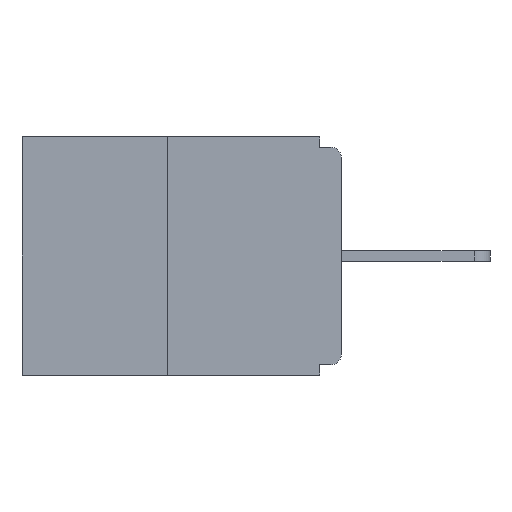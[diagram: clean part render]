
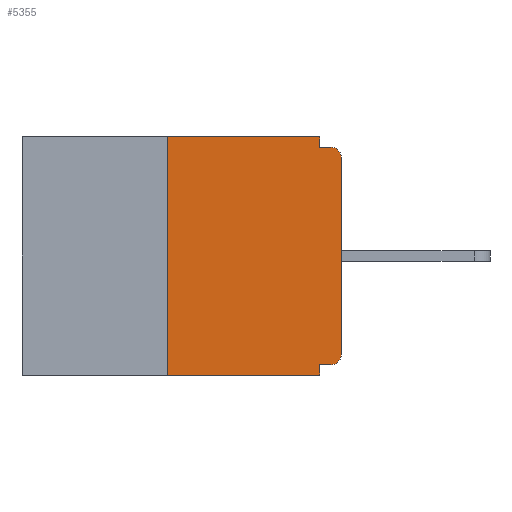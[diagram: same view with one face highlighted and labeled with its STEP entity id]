
A CAD part, left-side view. The second image highlights one B-rep face of the part: STEP entity #5355.
In plain terms, the highlighted planar face has unit normal (-1, 0, 0).
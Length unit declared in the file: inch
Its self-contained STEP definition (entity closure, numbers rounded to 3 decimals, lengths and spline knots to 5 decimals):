
#325 = ORIENTED_EDGE ( 'NONE', *, *, #5950, .T. ) ;
#400 = VERTEX_POINT ( 'NONE', #7091 ) ;
#432 = ORIENTED_EDGE ( 'NONE', *, *, #6960, .F. ) ;
#612 = AXIS2_PLACEMENT_3D ( 'NONE', #7975, #9048, #1179 ) ;
#764 = EDGE_CURVE ( 'NONE', #2450, #3988, #14203, .T. ) ;
#842 = VERTEX_POINT ( 'NONE', #9513 ) ;
#1100 = LINE ( 'NONE', #4835, #7129 ) ;
#1179 = DIRECTION ( 'NONE',  ( 0., 0., -1. ) ) ;
#1227 = DIRECTION ( 'NONE',  ( 0., -1., 0. ) ) ;
#1235 = EDGE_CURVE ( 'NONE', #7766, #1553, #11069, .T. ) ;
#1310 = LINE ( 'NONE', #10430, #7893 ) ;
#1400 = CARTESIAN_POINT ( 'NONE',  ( 0., 0., -0.328 ) ) ;
#1475 = EDGE_CURVE ( 'NONE', #2450, #7743, #1310, .T. ) ;
#1532 = CARTESIAN_POINT ( 'NONE',  ( 0., 0.46, 0. ) ) ;
#1553 = VERTEX_POINT ( 'NONE', #8556 ) ;
#1859 = CARTESIAN_POINT ( 'NONE',  ( 0., 0., -0.015 ) ) ;
#2295 = CARTESIAN_POINT ( 'NONE',  ( 0., 0., 0. ) ) ;
#2450 = VERTEX_POINT ( 'NONE', #4748 ) ;
#2460 = EDGE_CURVE ( 'NONE', #3988, #400, #8192, .T. ) ;
#2547 = DIRECTION ( 'NONE',  ( 0., -1., 0. ) ) ;
#3013 = DIRECTION ( 'NONE',  ( 0., -1., 0. ) ) ;
#3094 = EDGE_CURVE ( 'NONE', #842, #6810, #11705, .T. ) ;
#3638 = CARTESIAN_POINT ( 'NONE',  ( 0., 0.031, 0. ) ) ;
#3669 = VERTEX_POINT ( 'NONE', #6268 ) ;
#3782 = ORIENTED_EDGE ( 'NONE', *, *, #1235, .T. ) ;
#3988 = VERTEX_POINT ( 'NONE', #4119 ) ;
#4041 = CARTESIAN_POINT ( 'NONE',  ( 0., 0., -0.03 ) ) ;
#4119 = CARTESIAN_POINT ( 'NONE',  ( 0., 0.25, 0. ) ) ;
#4122 = VECTOR ( 'NONE', #5963, 39.37008 ) ;
#4569 = ORIENTED_EDGE ( 'NONE', *, *, #1475, .T. ) ;
#4748 = CARTESIAN_POINT ( 'NONE',  ( 0., 0.25, -0.343 ) ) ;
#4816 = DIRECTION ( 'NONE',  ( 0., 0., -1. ) ) ;
#4835 = CARTESIAN_POINT ( 'NONE',  ( 0., 0.031, -0.343 ) ) ;
#5017 = PLANE ( 'NONE',  #12383 ) ;
#5138 = CARTESIAN_POINT ( 'NONE',  ( 0., 0.031, -0.343 ) ) ;
#5355 = ADVANCED_FACE ( 'NONE', ( #11602 ), #5017, .F. ) ;
#5654 = CARTESIAN_POINT ( 'NONE',  ( 0., 0.25, 0. ) ) ;
#5797 = ORIENTED_EDGE ( 'NONE', *, *, #3094, .T. ) ;
#5883 = EDGE_CURVE ( 'NONE', #3669, #1553, #11937, .T. ) ;
#5950 = EDGE_CURVE ( 'NONE', #6810, #7766, #11747, .T. ) ;
#5963 = DIRECTION ( 'NONE',  ( 0., 1., 0. ) ) ;
#6045 = CARTESIAN_POINT ( 'NONE',  ( 0., 0.031, -0.328 ) ) ;
#6053 = DIRECTION ( 'NONE',  ( 0., 0., -1. ) ) ;
#6070 = VECTOR ( 'NONE', #1227, 39.37008 ) ;
#6083 = DIRECTION ( 'NONE',  ( 1., 0., 0. ) ) ;
#6204 = VERTEX_POINT ( 'NONE', #6045 ) ;
#6259 = CARTESIAN_POINT ( 'NONE',  ( 0., 0., -0.313 ) ) ;
#6268 = CARTESIAN_POINT ( 'NONE',  ( 0., 0.031, -0.015 ) ) ;
#6542 = DIRECTION ( 'NONE',  ( -1., 0., 0. ) ) ;
#6721 = ORIENTED_EDGE ( 'NONE', *, *, #6947, .F. ) ;
#6762 = VECTOR ( 'NONE', #7047, 39.37008 ) ;
#6810 = VERTEX_POINT ( 'NONE', #6259 ) ;
#6947 = EDGE_CURVE ( 'NONE', #400, #3669, #7843, .T. ) ;
#6960 = EDGE_CURVE ( 'NONE', #842, #6204, #9776, .T. ) ;
#7047 = DIRECTION ( 'NONE',  ( 0., 0., -1. ) ) ;
#7091 = CARTESIAN_POINT ( 'NONE',  ( 0., 0.031, 0. ) ) ;
#7129 = VECTOR ( 'NONE', #6053, 39.37008 ) ;
#7518 = VECTOR ( 'NONE', #11338, 39.37008 ) ;
#7741 = CARTESIAN_POINT ( 'NONE',  ( 0., 0.015, -0.313 ) ) ;
#7743 = VERTEX_POINT ( 'NONE', #5138 ) ;
#7766 = VERTEX_POINT ( 'NONE', #4041 ) ;
#7843 = LINE ( 'NONE', #3638, #6762 ) ;
#7861 = DIRECTION ( 'NONE',  ( 0., 0., 1. ) ) ;
#7893 = VECTOR ( 'NONE', #2547, 39.37008 ) ;
#7975 = CARTESIAN_POINT ( 'NONE',  ( 0., 0.015, -0.03 ) ) ;
#8027 = ORIENTED_EDGE ( 'NONE', *, *, #764, .F. ) ;
#8192 = LINE ( 'NONE', #13638, #6070 ) ;
#8485 = ORIENTED_EDGE ( 'NONE', *, *, #2460, .F. ) ;
#8556 = CARTESIAN_POINT ( 'NONE',  ( 0., 0.015, -0.015 ) ) ;
#9048 = DIRECTION ( 'NONE',  ( -1., 0., 0. ) ) ;
#9455 = VECTOR ( 'NONE', #3013, 39.37008 ) ;
#9513 = CARTESIAN_POINT ( 'NONE',  ( 0., 0.015, -0.328 ) ) ;
#9539 = AXIS2_PLACEMENT_3D ( 'NONE', #7741, #6542, #9905 ) ;
#9776 = LINE ( 'NONE', #1400, #4122 ) ;
#9905 = DIRECTION ( 'NONE',  ( 0., 0., -1. ) ) ;
#10430 = CARTESIAN_POINT ( 'NONE',  ( 0., 0.46, -0.343 ) ) ;
#11069 = CIRCLE ( 'NONE', #612, 0.015 ) ;
#11338 = DIRECTION ( 'NONE',  ( 0., 0., 1. ) ) ;
#11602 = FACE_OUTER_BOUND ( 'NONE', #12389, .T. ) ;
#11705 = CIRCLE ( 'NONE', #9539, 0.015 ) ;
#11747 = LINE ( 'NONE', #2295, #12275 ) ;
#11937 = LINE ( 'NONE', #1859, #9455 ) ;
#12275 = VECTOR ( 'NONE', #7861, 39.37008 ) ;
#12323 = ORIENTED_EDGE ( 'NONE', *, *, #14332, .F. ) ;
#12383 = AXIS2_PLACEMENT_3D ( 'NONE', #1532, #6083, #4816 ) ;
#12389 = EDGE_LOOP ( 'NONE', ( #8485, #8027, #4569, #12323, #432, #5797, #325, #3782, #13488, #6721 ) ) ;
#13488 = ORIENTED_EDGE ( 'NONE', *, *, #5883, .F. ) ;
#13638 = CARTESIAN_POINT ( 'NONE',  ( 0., 0.46, 0. ) ) ;
#14203 = LINE ( 'NONE', #5654, #7518 ) ;
#14332 = EDGE_CURVE ( 'NONE', #6204, #7743, #1100, .T. ) ;
